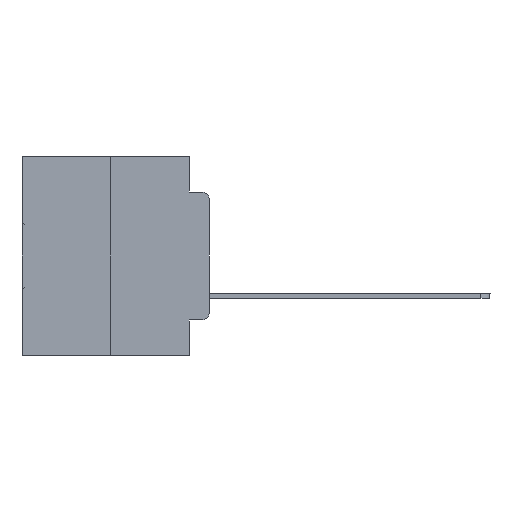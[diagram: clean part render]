
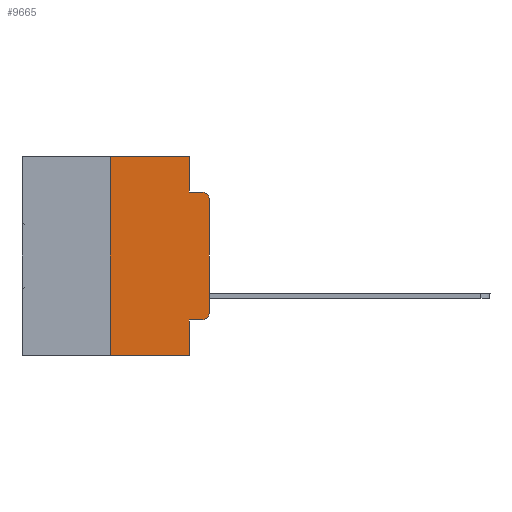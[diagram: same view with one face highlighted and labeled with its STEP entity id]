
A CAD part, left-side view. The second image highlights one B-rep face of the part: STEP entity #9665.
In plain terms, the highlighted planar face has unit normal (-1, 0, 0).
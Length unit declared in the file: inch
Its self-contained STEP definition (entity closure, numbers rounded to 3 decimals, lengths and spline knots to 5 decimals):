
#82 = EDGE_CURVE ( 'NONE', #23946, #10818, #16495, .T. ) ;
#449 = VECTOR ( 'NONE', #4058, 39.37008 ) ;
#997 = VECTOR ( 'NONE', #13852, 39.37008 ) ;
#1373 = EDGE_CURVE ( 'NONE', #2146, #27497, #6388, .T. ) ;
#2146 = VERTEX_POINT ( 'NONE', #32100 ) ;
#2417 = EDGE_CURVE ( 'NONE', #5460, #18055, #17505, .T. ) ;
#2775 = VECTOR ( 'NONE', #19272, 39.37008 ) ;
#2845 = CARTESIAN_POINT ( 'NONE',  ( 0., 0.051, 0. ) ) ;
#3888 = CARTESIAN_POINT ( 'NONE',  ( 0., 0., 0. ) ) ;
#4058 = DIRECTION ( 'NONE',  ( 0., -1., 0. ) ) ;
#4141 = VECTOR ( 'NONE', #20862, 39.37008 ) ;
#5460 = VERTEX_POINT ( 'NONE', #26244 ) ;
#6215 = EDGE_CURVE ( 'NONE', #9088, #20238, #11089, .T. ) ;
#6385 = AXIS2_PLACEMENT_3D ( 'NONE', #15612, #17748, #25447 ) ;
#6388 = LINE ( 'NONE', #21398, #29208 ) ;
#6564 = CARTESIAN_POINT ( 'NONE',  ( 0., 0.473, 0. ) ) ;
#6636 = VECTOR ( 'NONE', #17179, 39.37008 ) ;
#6715 = PLANE ( 'NONE',  #19883 ) ;
#7144 = CARTESIAN_POINT ( 'NONE',  ( 0., 0.02, -0.3915 ) ) ;
#7922 = VERTEX_POINT ( 'NONE', #10768 ) ;
#9088 = VERTEX_POINT ( 'NONE', #9789 ) ;
#9665 = ADVANCED_FACE ( 'NONE', ( #28464 ), #6715, .F. ) ;
#9789 = CARTESIAN_POINT ( 'NONE',  ( 0., 0., -0.3915 ) ) ;
#10018 = EDGE_CURVE ( 'NONE', #7922, #5460, #15501, .T. ) ;
#10768 = CARTESIAN_POINT ( 'NONE',  ( 0., 0.25, -0.5 ) ) ;
#10818 = VERTEX_POINT ( 'NONE', #15099 ) ;
#10839 = EDGE_CURVE ( 'NONE', #2146, #24406, #24780, .T. ) ;
#10968 = ORIENTED_EDGE ( 'NONE', *, *, #1373, .T. ) ;
#11089 = LINE ( 'NONE', #3888, #997 ) ;
#11316 = CARTESIAN_POINT ( 'NONE',  ( 0., 0.02, -0.4115 ) ) ;
#11462 = DIRECTION ( 'NONE',  ( 1., 0., 0. ) ) ;
#12327 = ORIENTED_EDGE ( 'NONE', *, *, #17614, .F. ) ;
#12616 = CARTESIAN_POINT ( 'NONE',  ( 0., 0.473, 0. ) ) ;
#13852 = DIRECTION ( 'NONE',  ( 0., 0., 1. ) ) ;
#14246 = EDGE_CURVE ( 'NONE', #27497, #9088, #26781, .T. ) ;
#15099 = CARTESIAN_POINT ( 'NONE',  ( 0., 0.02, -0.0885 ) ) ;
#15185 = CARTESIAN_POINT ( 'NONE',  ( 0., 0.25, 0. ) ) ;
#15279 = CARTESIAN_POINT ( 'NONE',  ( 0., 0.051, -0.0885 ) ) ;
#15357 = DIRECTION ( 'NONE',  ( 0., 0., 1. ) ) ;
#15501 = LINE ( 'NONE', #15185, #25126 ) ;
#15612 = CARTESIAN_POINT ( 'NONE',  ( 0., 0.02, -0.1085 ) ) ;
#16177 = DIRECTION ( 'NONE',  ( 0., -1., 0. ) ) ;
#16363 = DIRECTION ( 'NONE',  ( 0., 0., -1. ) ) ;
#16495 = LINE ( 'NONE', #24509, #2775 ) ;
#16801 = ORIENTED_EDGE ( 'NONE', *, *, #23211, .T. ) ;
#16990 = ORIENTED_EDGE ( 'NONE', *, *, #6215, .T. ) ;
#17179 = DIRECTION ( 'NONE',  ( 0., -1., 0. ) ) ;
#17505 = LINE ( 'NONE', #12616, #6636 ) ;
#17614 = EDGE_CURVE ( 'NONE', #18055, #23946, #23001, .T. ) ;
#17748 = DIRECTION ( 'NONE',  ( -1., 0., 0. ) ) ;
#18055 = VERTEX_POINT ( 'NONE', #28028 ) ;
#19272 = DIRECTION ( 'NONE',  ( 0., -1., 0. ) ) ;
#19726 = ORIENTED_EDGE ( 'NONE', *, *, #14246, .T. ) ;
#19883 = AXIS2_PLACEMENT_3D ( 'NONE', #6564, #11462, #16363 ) ;
#19978 = CARTESIAN_POINT ( 'NONE',  ( 0., 0.051, -0.5 ) ) ;
#20238 = VERTEX_POINT ( 'NONE', #30557 ) ;
#20862 = DIRECTION ( 'NONE',  ( 0., 0., -1. ) ) ;
#21398 = CARTESIAN_POINT ( 'NONE',  ( 0., 0.051, -0.4115 ) ) ;
#21521 = CIRCLE ( 'NONE', #6385, 0.02 ) ;
#22188 = EDGE_CURVE ( 'NONE', #20238, #10818, #21521, .T. ) ;
#23001 = LINE ( 'NONE', #30663, #4141 ) ;
#23211 = EDGE_CURVE ( 'NONE', #7922, #24406, #23850, .T. ) ;
#23463 = ORIENTED_EDGE ( 'NONE', *, *, #10839, .F. ) ;
#23703 = CARTESIAN_POINT ( 'NONE',  ( 0., 0.473, -0.5 ) ) ;
#23850 = LINE ( 'NONE', #23703, #449 ) ;
#23946 = VERTEX_POINT ( 'NONE', #15279 ) ;
#24166 = DIRECTION ( 'NONE',  ( 0., 0., -1. ) ) ;
#24406 = VERTEX_POINT ( 'NONE', #19978 ) ;
#24412 = EDGE_LOOP ( 'NONE', ( #16990, #27482, #24757, #12327, #30136, #29592, #16801, #23463, #10968, #19726 ) ) ;
#24509 = CARTESIAN_POINT ( 'NONE',  ( 0., 0.051, -0.0885 ) ) ;
#24757 = ORIENTED_EDGE ( 'NONE', *, *, #82, .F. ) ;
#24780 = LINE ( 'NONE', #2845, #26224 ) ;
#25096 = DIRECTION ( 'NONE',  ( 0., 0., -1. ) ) ;
#25126 = VECTOR ( 'NONE', #15357, 39.37008 ) ;
#25447 = DIRECTION ( 'NONE',  ( 0., 0., -1. ) ) ;
#26224 = VECTOR ( 'NONE', #25096, 39.37008 ) ;
#26244 = CARTESIAN_POINT ( 'NONE',  ( 0., 0.25, 0. ) ) ;
#26781 = CIRCLE ( 'NONE', #28332, 0.02 ) ;
#27482 = ORIENTED_EDGE ( 'NONE', *, *, #22188, .T. ) ;
#27497 = VERTEX_POINT ( 'NONE', #11316 ) ;
#28028 = CARTESIAN_POINT ( 'NONE',  ( 0., 0.051, 0. ) ) ;
#28332 = AXIS2_PLACEMENT_3D ( 'NONE', #7144, #29678, #24166 ) ;
#28464 = FACE_OUTER_BOUND ( 'NONE', #24412, .T. ) ;
#29208 = VECTOR ( 'NONE', #16177, 39.37008 ) ;
#29592 = ORIENTED_EDGE ( 'NONE', *, *, #10018, .F. ) ;
#29678 = DIRECTION ( 'NONE',  ( -1., 0., 0. ) ) ;
#30136 = ORIENTED_EDGE ( 'NONE', *, *, #2417, .F. ) ;
#30557 = CARTESIAN_POINT ( 'NONE',  ( 0., 0., -0.1085 ) ) ;
#30663 = CARTESIAN_POINT ( 'NONE',  ( 0., 0.051, 0. ) ) ;
#32100 = CARTESIAN_POINT ( 'NONE',  ( 0., 0.051, -0.4115 ) ) ;
